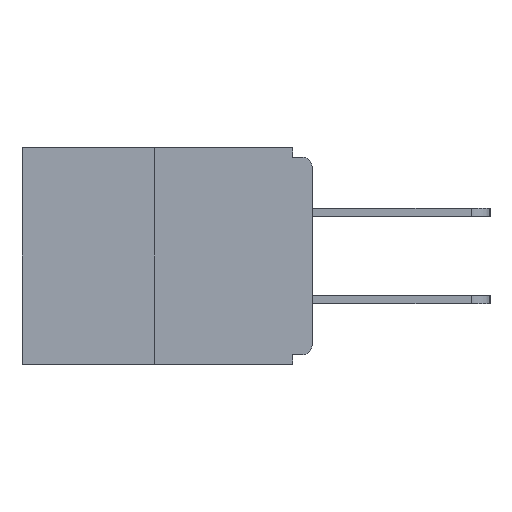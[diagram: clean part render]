
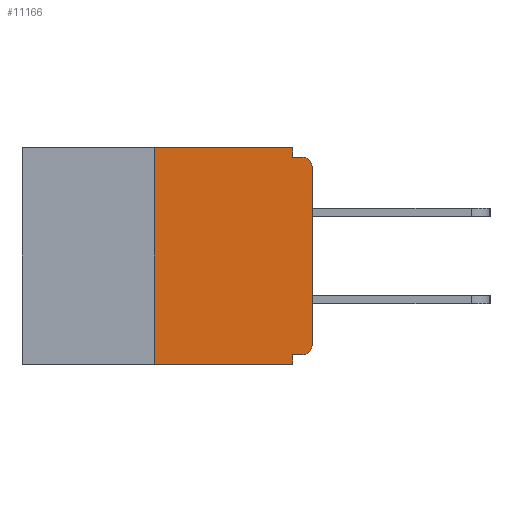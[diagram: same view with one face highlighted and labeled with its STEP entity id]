
A CAD part, left-side view. The second image highlights one B-rep face of the part: STEP entity #11166.
In plain terms, the highlighted planar face has unit normal (-1, 0, 0).
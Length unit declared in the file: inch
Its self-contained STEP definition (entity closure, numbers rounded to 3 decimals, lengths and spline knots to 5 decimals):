
#102 = ORIENTED_EDGE ( 'NONE', *, *, #23538, .F. ) ;
#339 = CARTESIAN_POINT ( 'NONE',  ( 0., 0.015, -0.328 ) ) ;
#772 = CARTESIAN_POINT ( 'NONE',  ( 0., 0.031, -0.015 ) ) ;
#983 = DIRECTION ( 'NONE',  ( 0., 0., 1. ) ) ;
#1235 = CIRCLE ( 'NONE', #20844, 0.015 ) ;
#1449 = FACE_OUTER_BOUND ( 'NONE', #2058, .T. ) ;
#1454 = CARTESIAN_POINT ( 'NONE',  ( 0., 0.031, -0.328 ) ) ;
#1578 = PLANE ( 'NONE',  #17385 ) ;
#1803 = CARTESIAN_POINT ( 'NONE',  ( 0., 0.25, 0. ) ) ;
#2058 = EDGE_LOOP ( 'NONE', ( #18305, #9097, #18070, #6816, #17333, #14431, #3567, #10513, #5922, #102 ) ) ;
#2436 = DIRECTION ( 'NONE',  ( 0., -1., 0. ) ) ;
#3167 = VERTEX_POINT ( 'NONE', #339 ) ;
#3382 = CARTESIAN_POINT ( 'NONE',  ( 0., 0., -0.313 ) ) ;
#3386 = DIRECTION ( 'NONE',  ( 1., 0., 0. ) ) ;
#3475 = LINE ( 'NONE', #20325, #11417 ) ;
#3567 = ORIENTED_EDGE ( 'NONE', *, *, #16075, .T. ) ;
#3667 = VECTOR ( 'NONE', #983, 39.37008 ) ;
#3858 = LINE ( 'NONE', #18355, #15330 ) ;
#4242 = LINE ( 'NONE', #11620, #6575 ) ;
#5028 = VECTOR ( 'NONE', #14708, 39.37008 ) ;
#5852 = CARTESIAN_POINT ( 'NONE',  ( 0., 0.25, 0. ) ) ;
#5922 = ORIENTED_EDGE ( 'NONE', *, *, #23479, .F. ) ;
#6159 = CARTESIAN_POINT ( 'NONE',  ( 0., 0.25, -0.343 ) ) ;
#6263 = LINE ( 'NONE', #9541, #11882 ) ;
#6575 = VECTOR ( 'NONE', #2436, 39.37008 ) ;
#6775 = DIRECTION ( 'NONE',  ( -1., 0., 0. ) ) ;
#6816 = ORIENTED_EDGE ( 'NONE', *, *, #19973, .F. ) ;
#7110 = CARTESIAN_POINT ( 'NONE',  ( 0., 0.46, 0. ) ) ;
#7742 = CARTESIAN_POINT ( 'NONE',  ( 0., 0., -0.03 ) ) ;
#8076 = AXIS2_PLACEMENT_3D ( 'NONE', #14472, #14959, #14722 ) ;
#8816 = CARTESIAN_POINT ( 'NONE',  ( 0., 0.46, 0. ) ) ;
#9005 = EDGE_CURVE ( 'NONE', #23408, #15252, #12783, .T. ) ;
#9097 = ORIENTED_EDGE ( 'NONE', *, *, #13772, .F. ) ;
#9266 = DIRECTION ( 'NONE',  ( 0., 1., 0. ) ) ;
#9541 = CARTESIAN_POINT ( 'NONE',  ( 0., 0.031, 0. ) ) ;
#9642 = VERTEX_POINT ( 'NONE', #7742 ) ;
#9652 = EDGE_CURVE ( 'NONE', #9754, #13016, #4242, .T. ) ;
#9754 = VERTEX_POINT ( 'NONE', #6159 ) ;
#9771 = VECTOR ( 'NONE', #22614, 39.37008 ) ;
#9822 = CARTESIAN_POINT ( 'NONE',  ( 0., 0., 0. ) ) ;
#9853 = VERTEX_POINT ( 'NONE', #3382 ) ;
#10440 = CIRCLE ( 'NONE', #8076, 0.015 ) ;
#10443 = VERTEX_POINT ( 'NONE', #772 ) ;
#10513 = ORIENTED_EDGE ( 'NONE', *, *, #12430, .T. ) ;
#10623 = CARTESIAN_POINT ( 'NONE',  ( 0., 0.031, 0. ) ) ;
#10879 = CARTESIAN_POINT ( 'NONE',  ( 0., 0.031, -0.343 ) ) ;
#11166 = ADVANCED_FACE ( 'NONE', ( #1449 ), #1578, .F. ) ;
#11417 = VECTOR ( 'NONE', #9266, 39.37008 ) ;
#11422 = CARTESIAN_POINT ( 'NONE',  ( 0., 0.015, -0.015 ) ) ;
#11620 = CARTESIAN_POINT ( 'NONE',  ( 0., 0.46, -0.343 ) ) ;
#11882 = VECTOR ( 'NONE', #22659, 39.37008 ) ;
#12430 = EDGE_CURVE ( 'NONE', #9642, #19312, #1235, .T. ) ;
#12783 = LINE ( 'NONE', #7110, #5028 ) ;
#13016 = VERTEX_POINT ( 'NONE', #22631 ) ;
#13772 = EDGE_CURVE ( 'NONE', #9754, #23408, #15040, .T. ) ;
#13890 = LINE ( 'NONE', #9822, #3667 ) ;
#14431 = ORIENTED_EDGE ( 'NONE', *, *, #15055, .T. ) ;
#14472 = CARTESIAN_POINT ( 'NONE',  ( 0., 0.015, -0.313 ) ) ;
#14708 = DIRECTION ( 'NONE',  ( 0., -1., 0. ) ) ;
#14722 = DIRECTION ( 'NONE',  ( 0., 0., -1. ) ) ;
#14959 = DIRECTION ( 'NONE',  ( -1., 0., 0. ) ) ;
#15040 = LINE ( 'NONE', #5852, #9771 ) ;
#15055 = EDGE_CURVE ( 'NONE', #3167, #9853, #10440, .T. ) ;
#15252 = VERTEX_POINT ( 'NONE', #10623 ) ;
#15330 = VECTOR ( 'NONE', #20244, 39.37008 ) ;
#16075 = EDGE_CURVE ( 'NONE', #9853, #9642, #13890, .T. ) ;
#16814 = EDGE_CURVE ( 'NONE', #3167, #23333, #3475, .T. ) ;
#17333 = ORIENTED_EDGE ( 'NONE', *, *, #16814, .F. ) ;
#17385 = AXIS2_PLACEMENT_3D ( 'NONE', #8816, #3386, #17898 ) ;
#17898 = DIRECTION ( 'NONE',  ( 0., 0., -1. ) ) ;
#18070 = ORIENTED_EDGE ( 'NONE', *, *, #9652, .T. ) ;
#18305 = ORIENTED_EDGE ( 'NONE', *, *, #9005, .F. ) ;
#18355 = CARTESIAN_POINT ( 'NONE',  ( 0., 0., -0.015 ) ) ;
#19312 = VERTEX_POINT ( 'NONE', #11422 ) ;
#19541 = LINE ( 'NONE', #10879, #22669 ) ;
#19677 = DIRECTION ( 'NONE',  ( 0., 0., -1. ) ) ;
#19973 = EDGE_CURVE ( 'NONE', #23333, #13016, #19541, .T. ) ;
#20244 = DIRECTION ( 'NONE',  ( 0., -1., 0. ) ) ;
#20325 = CARTESIAN_POINT ( 'NONE',  ( 0., 0., -0.328 ) ) ;
#20844 = AXIS2_PLACEMENT_3D ( 'NONE', #23299, #6775, #19677 ) ;
#21595 = DIRECTION ( 'NONE',  ( 0., 0., -1. ) ) ;
#22614 = DIRECTION ( 'NONE',  ( 0., 0., 1. ) ) ;
#22631 = CARTESIAN_POINT ( 'NONE',  ( 0., 0.031, -0.343 ) ) ;
#22659 = DIRECTION ( 'NONE',  ( 0., 0., -1. ) ) ;
#22669 = VECTOR ( 'NONE', #21595, 39.37008 ) ;
#23299 = CARTESIAN_POINT ( 'NONE',  ( 0., 0.015, -0.03 ) ) ;
#23333 = VERTEX_POINT ( 'NONE', #1454 ) ;
#23408 = VERTEX_POINT ( 'NONE', #1803 ) ;
#23479 = EDGE_CURVE ( 'NONE', #10443, #19312, #3858, .T. ) ;
#23538 = EDGE_CURVE ( 'NONE', #15252, #10443, #6263, .T. ) ;
